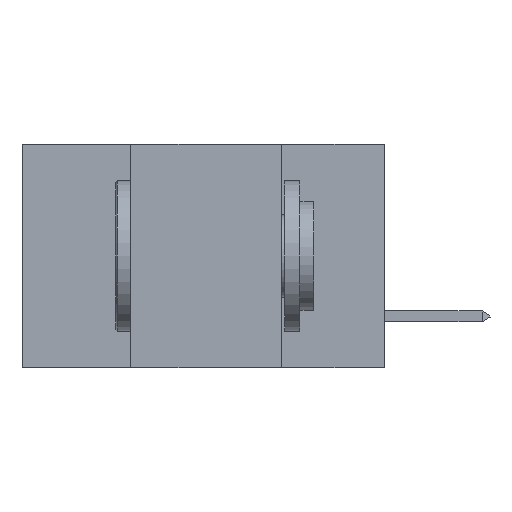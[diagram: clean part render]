
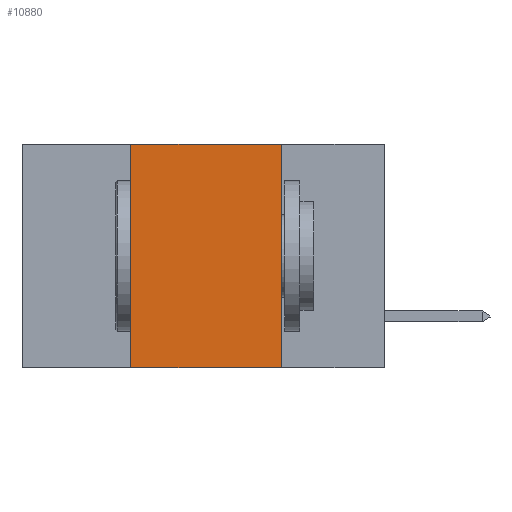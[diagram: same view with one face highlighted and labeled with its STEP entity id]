
A CAD part, left-side view. The second image highlights one B-rep face of the part: STEP entity #10880.
In plain terms, the highlighted planar face has unit normal (-1, 0, 0).
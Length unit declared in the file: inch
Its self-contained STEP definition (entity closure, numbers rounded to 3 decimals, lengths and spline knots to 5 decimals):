
#244 = VERTEX_POINT ( 'NONE', #6123 ) ;
#447 = FACE_OUTER_BOUND ( 'NONE', #11852, .T. ) ;
#1512 = DIRECTION ( 'NONE',  ( 0., -1., 0. ) ) ;
#1900 = VECTOR ( 'NONE', #1512, 39.37008 ) ;
#2119 = EDGE_CURVE ( 'NONE', #8186, #244, #8438, .T. ) ;
#2232 = CARTESIAN_POINT ( 'NONE',  ( 0., 0.17, 0. ) ) ;
#3278 = DIRECTION ( 'NONE',  ( 0., 0., -1. ) ) ;
#3417 = CARTESIAN_POINT ( 'NONE',  ( 0., 0.6, 0. ) ) ;
#3695 = CARTESIAN_POINT ( 'NONE',  ( 0., 0.42, 0. ) ) ;
#4356 = DIRECTION ( 'NONE',  ( 0., 0., -1. ) ) ;
#4808 = LINE ( 'NONE', #6357, #1900 ) ;
#4836 = CARTESIAN_POINT ( 'NONE',  ( 0., 0.42, 0. ) ) ;
#5107 = CARTESIAN_POINT ( 'NONE',  ( 0., 0.42, -0.37 ) ) ;
#5343 = VECTOR ( 'NONE', #7274, 39.37008 ) ;
#5826 = VERTEX_POINT ( 'NONE', #9823 ) ;
#6123 = CARTESIAN_POINT ( 'NONE',  ( 0., 0.17, -0.37 ) ) ;
#6309 = VECTOR ( 'NONE', #9256, 39.37008 ) ;
#6357 = CARTESIAN_POINT ( 'NONE',  ( 0., 0.6, 0. ) ) ;
#6871 = VECTOR ( 'NONE', #3278, 39.37008 ) ;
#7274 = DIRECTION ( 'NONE',  ( 0., -1., 0. ) ) ;
#7407 = ORIENTED_EDGE ( 'NONE', *, *, #9693, .F. ) ;
#7449 = ORIENTED_EDGE ( 'NONE', *, *, #9858, .F. ) ;
#7564 = ORIENTED_EDGE ( 'NONE', *, *, #8480, .F. ) ;
#7606 = CARTESIAN_POINT ( 'NONE',  ( 0., 0.6, -0.37 ) ) ;
#7826 = ORIENTED_EDGE ( 'NONE', *, *, #2119, .T. ) ;
#7994 = VERTEX_POINT ( 'NONE', #4836 ) ;
#8186 = VERTEX_POINT ( 'NONE', #5107 ) ;
#8438 = LINE ( 'NONE', #7606, #5343 ) ;
#8480 = EDGE_CURVE ( 'NONE', #8186, #7994, #11350, .T. ) ;
#8994 = PLANE ( 'NONE',  #10183 ) ;
#9256 = DIRECTION ( 'NONE',  ( 0., 0., 1. ) ) ;
#9693 = EDGE_CURVE ( 'NONE', #5826, #244, #11318, .T. ) ;
#9823 = CARTESIAN_POINT ( 'NONE',  ( 0., 0.17, 0. ) ) ;
#9858 = EDGE_CURVE ( 'NONE', #7994, #5826, #4808, .T. ) ;
#9869 = DIRECTION ( 'NONE',  ( 1., 0., 0. ) ) ;
#10183 = AXIS2_PLACEMENT_3D ( 'NONE', #3417, #9869, #4356 ) ;
#10880 = ADVANCED_FACE ( 'NONE', ( #447 ), #8994, .F. ) ;
#11318 = LINE ( 'NONE', #2232, #6871 ) ;
#11350 = LINE ( 'NONE', #3695, #6309 ) ;
#11852 = EDGE_LOOP ( 'NONE', ( #7407, #7449, #7564, #7826 ) ) ;
